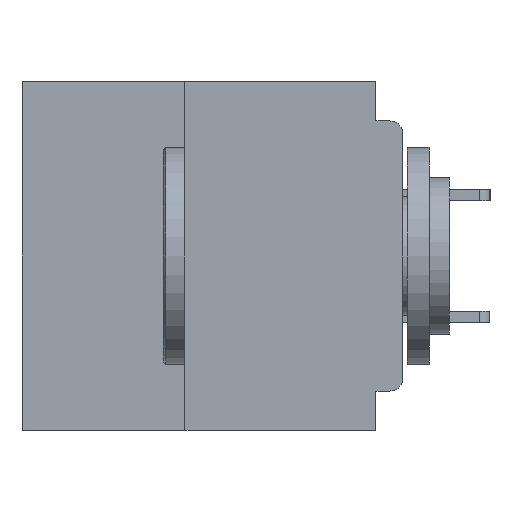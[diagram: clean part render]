
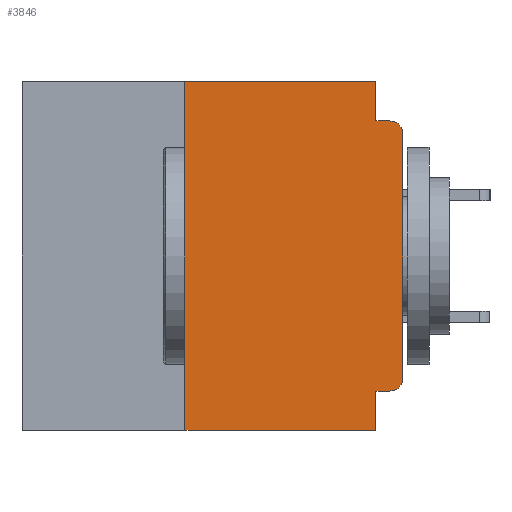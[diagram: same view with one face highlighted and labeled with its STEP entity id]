
A CAD part, left-side view. The second image highlights one B-rep face of the part: STEP entity #3846.
In plain terms, the highlighted planar face has unit normal (-1, 0, 0).
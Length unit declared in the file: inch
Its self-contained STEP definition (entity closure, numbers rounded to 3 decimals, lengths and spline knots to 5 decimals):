
#1063 = CIRCLE ( 'NONE', #44784, 0.015 ) ;
#1584 = ORIENTED_EDGE ( 'NONE', *, *, #54727, .F. ) ;
#2466 = DIRECTION ( 'NONE',  ( -1., 0., 0. ) ) ;
#2973 = VECTOR ( 'NONE', #7237, 39.37008 ) ;
#3011 = CARTESIAN_POINT ( 'NONE',  ( 0., 0.031, -0.4 ) ) ;
#3139 = AXIS2_PLACEMENT_3D ( 'NONE', #27408, #59829, #32094 ) ;
#3846 = ADVANCED_FACE ( 'NONE', ( #26298 ), #36628, .F. ) ;
#3939 = EDGE_CURVE ( 'NONE', #35430, #36248, #31412, .T. ) ;
#4333 = CARTESIAN_POINT ( 'NONE',  ( 0., 0., -0.355 ) ) ;
#4886 = CARTESIAN_POINT ( 'NONE',  ( 0., 0.25, -0.4 ) ) ;
#5987 = VECTOR ( 'NONE', #41532, 39.37008 ) ;
#6982 = VERTEX_POINT ( 'NONE', #53792 ) ;
#7237 = DIRECTION ( 'NONE',  ( 0., -1., 0. ) ) ;
#7451 = LINE ( 'NONE', #60074, #5987 ) ;
#7758 = DIRECTION ( 'NONE',  ( 0., 0., -1. ) ) ;
#8807 = ORIENTED_EDGE ( 'NONE', *, *, #3939, .T. ) ;
#10008 = EDGE_CURVE ( 'NONE', #18853, #6982, #16929, .T. ) ;
#10098 = CARTESIAN_POINT ( 'NONE',  ( 0., 0.015, -0.045 ) ) ;
#10631 = CARTESIAN_POINT ( 'NONE',  ( 0., 0.25, -0.4 ) ) ;
#11731 = VECTOR ( 'NONE', #7758, 39.37008 ) ;
#11956 = CARTESIAN_POINT ( 'NONE',  ( 0., 0.437, 0. ) ) ;
#13808 = CARTESIAN_POINT ( 'NONE',  ( 0., 0.437, -0.4 ) ) ;
#14980 = EDGE_CURVE ( 'NONE', #22459, #56472, #7451, .T. ) ;
#15566 = CARTESIAN_POINT ( 'NONE',  ( 0., 0.25, 0. ) ) ;
#15899 = LINE ( 'NONE', #27003, #39432 ) ;
#16504 = CARTESIAN_POINT ( 'NONE',  ( 0., 0.015, -0.355 ) ) ;
#16886 = EDGE_CURVE ( 'NONE', #33737, #30234, #59034, .T. ) ;
#16929 = LINE ( 'NONE', #11956, #2973 ) ;
#17900 = DIRECTION ( 'NONE',  ( 1., 0., 0. ) ) ;
#18227 = CARTESIAN_POINT ( 'NONE',  ( 0., 0.031, 0. ) ) ;
#18767 = VECTOR ( 'NONE', #41852, 39.37008 ) ;
#18853 = VERTEX_POINT ( 'NONE', #15566 ) ;
#19071 = EDGE_CURVE ( 'NONE', #30234, #36248, #49079, .T. ) ;
#20031 = ORIENTED_EDGE ( 'NONE', *, *, #58144, .T. ) ;
#22459 = VERTEX_POINT ( 'NONE', #46424 ) ;
#25369 = VERTEX_POINT ( 'NONE', #55265 ) ;
#25460 = ORIENTED_EDGE ( 'NONE', *, *, #14980, .F. ) ;
#26298 = FACE_OUTER_BOUND ( 'NONE', #56359, .T. ) ;
#27003 = CARTESIAN_POINT ( 'NONE',  ( 0., 0., 0. ) ) ;
#27074 = EDGE_CURVE ( 'NONE', #33737, #25369, #1063, .T. ) ;
#27094 = VERTEX_POINT ( 'NONE', #44563 ) ;
#27243 = CARTESIAN_POINT ( 'NONE',  ( 0., 0.437, 0. ) ) ;
#27408 = CARTESIAN_POINT ( 'NONE',  ( 0., 0.015, -0.06 ) ) ;
#29544 = ORIENTED_EDGE ( 'NONE', *, *, #16886, .F. ) ;
#30234 = VERTEX_POINT ( 'NONE', #34182 ) ;
#30309 = ORIENTED_EDGE ( 'NONE', *, *, #10008, .F. ) ;
#30688 = CARTESIAN_POINT ( 'NONE',  ( 0., 0.015, -0.34 ) ) ;
#31412 = LINE ( 'NONE', #13808, #42382 ) ;
#32011 = VECTOR ( 'NONE', #43476, 39.37008 ) ;
#32094 = DIRECTION ( 'NONE',  ( 0., 0., -1. ) ) ;
#32538 = DIRECTION ( 'NONE',  ( 0., 1., 0. ) ) ;
#33171 = ORIENTED_EDGE ( 'NONE', *, *, #19071, .F. ) ;
#33737 = VERTEX_POINT ( 'NONE', #16504 ) ;
#33819 = CARTESIAN_POINT ( 'NONE',  ( 0., 0.031, -0.4 ) ) ;
#34182 = CARTESIAN_POINT ( 'NONE',  ( 0., 0.031, -0.355 ) ) ;
#35365 = DIRECTION ( 'NONE',  ( 0., 0., -1. ) ) ;
#35430 = VERTEX_POINT ( 'NONE', #4886 ) ;
#35878 = VECTOR ( 'NONE', #32538, 39.37008 ) ;
#36248 = VERTEX_POINT ( 'NONE', #33819 ) ;
#36628 = PLANE ( 'NONE',  #48657 ) ;
#37431 = DIRECTION ( 'NONE',  ( 0., -1., 0. ) ) ;
#39432 = VECTOR ( 'NONE', #55001, 39.37008 ) ;
#40662 = EDGE_CURVE ( 'NONE', #27094, #56472, #48782, .T. ) ;
#40665 = ORIENTED_EDGE ( 'NONE', *, *, #40662, .T. ) ;
#41532 = DIRECTION ( 'NONE',  ( 0., -1., 0. ) ) ;
#41852 = DIRECTION ( 'NONE',  ( 0., 0., -1. ) ) ;
#42382 = VECTOR ( 'NONE', #37431, 39.37008 ) ;
#43476 = DIRECTION ( 'NONE',  ( 0., 0., 1. ) ) ;
#44427 = LINE ( 'NONE', #10631, #32011 ) ;
#44563 = CARTESIAN_POINT ( 'NONE',  ( 0., 0., -0.06 ) ) ;
#44784 = AXIS2_PLACEMENT_3D ( 'NONE', #30688, #2466, #35365 ) ;
#45338 = ORIENTED_EDGE ( 'NONE', *, *, #54533, .F. ) ;
#46424 = CARTESIAN_POINT ( 'NONE',  ( 0., 0.031, -0.045 ) ) ;
#48657 = AXIS2_PLACEMENT_3D ( 'NONE', #27243, #17900, #50618 ) ;
#48782 = CIRCLE ( 'NONE', #3139, 0.015 ) ;
#49079 = LINE ( 'NONE', #3011, #11731 ) ;
#50618 = DIRECTION ( 'NONE',  ( 0., 0., -1. ) ) ;
#53792 = CARTESIAN_POINT ( 'NONE',  ( 0., 0.031, 0. ) ) ;
#54533 = EDGE_CURVE ( 'NONE', #6982, #22459, #57440, .T. ) ;
#54727 = EDGE_CURVE ( 'NONE', #35430, #18853, #44427, .T. ) ;
#55001 = DIRECTION ( 'NONE',  ( 0., 0., 1. ) ) ;
#55022 = ORIENTED_EDGE ( 'NONE', *, *, #27074, .T. ) ;
#55265 = CARTESIAN_POINT ( 'NONE',  ( 0., 0., -0.34 ) ) ;
#56359 = EDGE_LOOP ( 'NONE', ( #20031, #40665, #25460, #45338, #30309, #1584, #8807, #33171, #29544, #55022 ) ) ;
#56472 = VERTEX_POINT ( 'NONE', #10098 ) ;
#57440 = LINE ( 'NONE', #18227, #18767 ) ;
#58144 = EDGE_CURVE ( 'NONE', #25369, #27094, #15899, .T. ) ;
#59034 = LINE ( 'NONE', #4333, #35878 ) ;
#59829 = DIRECTION ( 'NONE',  ( -1., 0., 0. ) ) ;
#60074 = CARTESIAN_POINT ( 'NONE',  ( 0., 0., -0.045 ) ) ;
